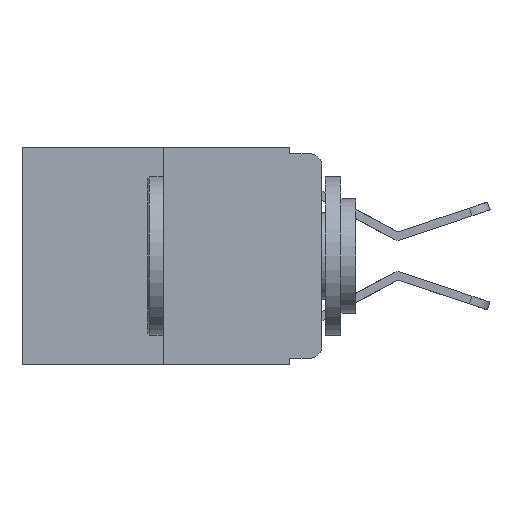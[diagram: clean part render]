
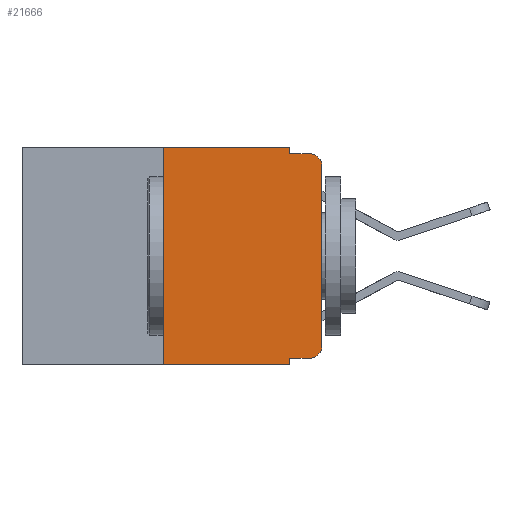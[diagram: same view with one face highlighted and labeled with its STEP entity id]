
A CAD part, left-side view. The second image highlights one B-rep face of the part: STEP entity #21666.
In plain terms, the highlighted planar face has unit normal (-1, 0, 0).
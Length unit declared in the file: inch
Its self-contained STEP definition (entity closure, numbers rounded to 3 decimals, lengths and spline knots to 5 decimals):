
#51 = ORIENTED_EDGE ( 'NONE', *, *, #12395, .T. ) ;
#410 = DIRECTION ( 'NONE',  ( 0., 0., -1. ) ) ;
#664 = ORIENTED_EDGE ( 'NONE', *, *, #10391, .T. ) ;
#2895 = AXIS2_PLACEMENT_3D ( 'NONE', #8695, #10587, #23767 ) ;
#4017 = DIRECTION ( 'NONE',  ( 0., -1., 0. ) ) ;
#4125 = VECTOR ( 'NONE', #14972, 39.37008 ) ;
#4153 = VERTEX_POINT ( 'NONE', #19864 ) ;
#4266 = FACE_OUTER_BOUND ( 'NONE', #15460, .T. ) ;
#4393 = LINE ( 'NONE', #5060, #18406 ) ;
#4867 = DIRECTION ( 'NONE',  ( 0., 0., -1. ) ) ;
#5060 = CARTESIAN_POINT ( 'NONE',  ( 0., 0.051, -0.01 ) ) ;
#5384 = VERTEX_POINT ( 'NONE', #20898 ) ;
#5825 = CARTESIAN_POINT ( 'NONE',  ( 0., 0.473, -0.343 ) ) ;
#5830 = VERTEX_POINT ( 'NONE', #20952 ) ;
#5960 = CARTESIAN_POINT ( 'NONE',  ( 0., 0.051, -0.343 ) ) ;
#6520 = ORIENTED_EDGE ( 'NONE', *, *, #17463, .F. ) ;
#6809 = ORIENTED_EDGE ( 'NONE', *, *, #20420, .T. ) ;
#6834 = CARTESIAN_POINT ( 'NONE',  ( 0., 0.051, 0. ) ) ;
#6900 = DIRECTION ( 'NONE',  ( 0., 0., 1. ) ) ;
#7329 = AXIS2_PLACEMENT_3D ( 'NONE', #23294, #12032, #410 ) ;
#7414 = ORIENTED_EDGE ( 'NONE', *, *, #12076, .F. ) ;
#8255 = EDGE_CURVE ( 'NONE', #5384, #19410, #18813, .T. ) ;
#8486 = DIRECTION ( 'NONE',  ( -1., 0., 0. ) ) ;
#8572 = EDGE_CURVE ( 'NONE', #5830, #16309, #12336, .T. ) ;
#8695 = CARTESIAN_POINT ( 'NONE',  ( 0., 0.473, 0. ) ) ;
#8768 = VECTOR ( 'NONE', #16850, 39.37008 ) ;
#9230 = AXIS2_PLACEMENT_3D ( 'NONE', #19781, #8486, #21675 ) ;
#9276 = LINE ( 'NONE', #16803, #4125 ) ;
#9373 = EDGE_CURVE ( 'NONE', #16309, #16757, #15316, .T. ) ;
#9966 = CARTESIAN_POINT ( 'NONE',  ( 0., 0.473, 0. ) ) ;
#10391 = EDGE_CURVE ( 'NONE', #19692, #22056, #21713, .T. ) ;
#10587 = DIRECTION ( 'NONE',  ( 1., 0., 0. ) ) ;
#11295 = VERTEX_POINT ( 'NONE', #16210 ) ;
#11511 = LINE ( 'NONE', #9966, #14190 ) ;
#12032 = DIRECTION ( 'NONE',  ( -1., 0., 0. ) ) ;
#12076 = EDGE_CURVE ( 'NONE', #19410, #19331, #4393, .T. ) ;
#12336 = CIRCLE ( 'NONE', #7329, 0.02 ) ;
#12395 = EDGE_CURVE ( 'NONE', #11295, #5830, #12500, .T. ) ;
#12439 = PLANE ( 'NONE',  #2895 ) ;
#12500 = LINE ( 'NONE', #15498, #22486 ) ;
#13044 = CARTESIAN_POINT ( 'NONE',  ( 0., 0.051, 0. ) ) ;
#14190 = VECTOR ( 'NONE', #15694, 39.37008 ) ;
#14668 = EDGE_CURVE ( 'NONE', #4153, #5384, #11511, .T. ) ;
#14800 = CARTESIAN_POINT ( 'NONE',  ( 0., 0., -0.313 ) ) ;
#14972 = DIRECTION ( 'NONE',  ( 0., 0., 1. ) ) ;
#15316 = LINE ( 'NONE', #18264, #19696 ) ;
#15460 = EDGE_LOOP ( 'NONE', ( #15728, #6809, #7414, #23072, #24239, #19836, #664, #6520, #51, #21599 ) ) ;
#15498 = CARTESIAN_POINT ( 'NONE',  ( 0., 0.051, -0.333 ) ) ;
#15694 = DIRECTION ( 'NONE',  ( 0., -1., 0. ) ) ;
#15728 = ORIENTED_EDGE ( 'NONE', *, *, #9373, .T. ) ;
#16210 = CARTESIAN_POINT ( 'NONE',  ( 0., 0.051, -0.333 ) ) ;
#16309 = VERTEX_POINT ( 'NONE', #14800 ) ;
#16757 = VERTEX_POINT ( 'NONE', #19925 ) ;
#16803 = CARTESIAN_POINT ( 'NONE',  ( 0., 0.25, 0. ) ) ;
#16850 = DIRECTION ( 'NONE',  ( 0., 0., -1. ) ) ;
#17242 = DIRECTION ( 'NONE',  ( 0., -1., 0. ) ) ;
#17463 = EDGE_CURVE ( 'NONE', #11295, #22056, #19616, .T. ) ;
#17626 = EDGE_CURVE ( 'NONE', #19692, #4153, #9276, .T. ) ;
#18264 = CARTESIAN_POINT ( 'NONE',  ( 0., 0., 0. ) ) ;
#18406 = VECTOR ( 'NONE', #20240, 39.37008 ) ;
#18609 = CARTESIAN_POINT ( 'NONE',  ( 0., 0.051, -0.01 ) ) ;
#18813 = LINE ( 'NONE', #13044, #8768 ) ;
#19331 = VERTEX_POINT ( 'NONE', #24017 ) ;
#19410 = VERTEX_POINT ( 'NONE', #18609 ) ;
#19490 = CARTESIAN_POINT ( 'NONE',  ( 0., 0.25, -0.343 ) ) ;
#19616 = LINE ( 'NONE', #6834, #23441 ) ;
#19692 = VERTEX_POINT ( 'NONE', #19490 ) ;
#19696 = VECTOR ( 'NONE', #6900, 39.37008 ) ;
#19781 = CARTESIAN_POINT ( 'NONE',  ( 0., 0.02, -0.03 ) ) ;
#19836 = ORIENTED_EDGE ( 'NONE', *, *, #17626, .F. ) ;
#19864 = CARTESIAN_POINT ( 'NONE',  ( 0., 0.25, 0. ) ) ;
#19925 = CARTESIAN_POINT ( 'NONE',  ( 0., 0., -0.03 ) ) ;
#20240 = DIRECTION ( 'NONE',  ( 0., -1., 0. ) ) ;
#20420 = EDGE_CURVE ( 'NONE', #16757, #19331, #21795, .T. ) ;
#20898 = CARTESIAN_POINT ( 'NONE',  ( 0., 0.051, 0. ) ) ;
#20952 = CARTESIAN_POINT ( 'NONE',  ( 0., 0.02, -0.333 ) ) ;
#21599 = ORIENTED_EDGE ( 'NONE', *, *, #8572, .T. ) ;
#21666 = ADVANCED_FACE ( 'NONE', ( #4266 ), #12439, .F. ) ;
#21675 = DIRECTION ( 'NONE',  ( 0., 0., -1. ) ) ;
#21713 = LINE ( 'NONE', #5825, #22890 ) ;
#21795 = CIRCLE ( 'NONE', #9230, 0.02 ) ;
#22056 = VERTEX_POINT ( 'NONE', #5960 ) ;
#22486 = VECTOR ( 'NONE', #4017, 39.37008 ) ;
#22890 = VECTOR ( 'NONE', #17242, 39.37008 ) ;
#23072 = ORIENTED_EDGE ( 'NONE', *, *, #8255, .F. ) ;
#23294 = CARTESIAN_POINT ( 'NONE',  ( 0., 0.02, -0.313 ) ) ;
#23441 = VECTOR ( 'NONE', #4867, 39.37008 ) ;
#23767 = DIRECTION ( 'NONE',  ( 0., 0., -1. ) ) ;
#24017 = CARTESIAN_POINT ( 'NONE',  ( 0., 0.02, -0.01 ) ) ;
#24239 = ORIENTED_EDGE ( 'NONE', *, *, #14668, .F. ) ;
